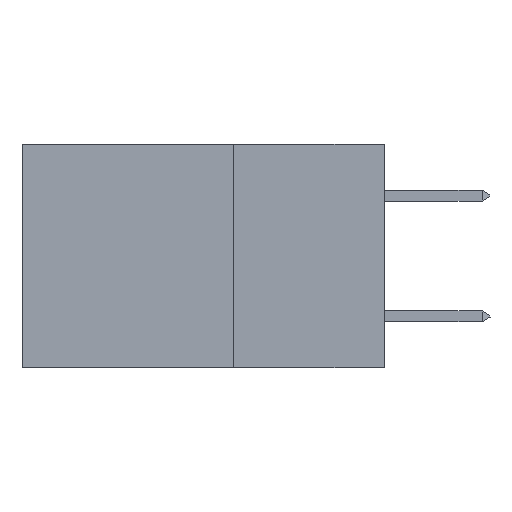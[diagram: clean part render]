
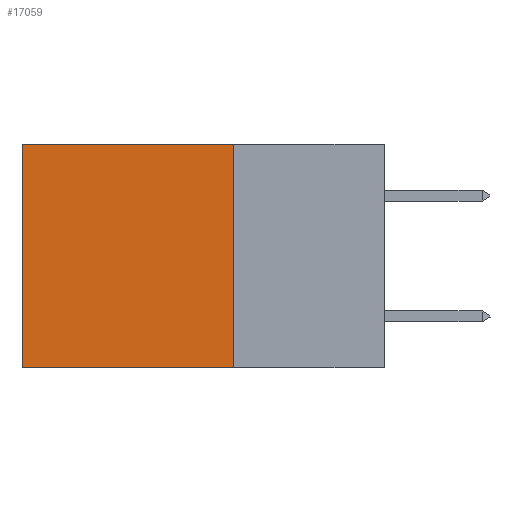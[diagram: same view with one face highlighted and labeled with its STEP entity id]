
A CAD part, left-side view. The second image highlights one B-rep face of the part: STEP entity #17059.
In plain terms, the highlighted planar face has unit normal (-1, 0, 0).
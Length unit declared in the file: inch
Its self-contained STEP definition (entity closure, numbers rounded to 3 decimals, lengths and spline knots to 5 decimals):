
#286 = VECTOR ( 'NONE', #23873, 39.37008 ) ;
#398 = CARTESIAN_POINT ( 'NONE',  ( 0.2875, 0.25, -0.37 ) ) ;
#1246 = CARTESIAN_POINT ( 'NONE',  ( 0.2875, 0.25, 0. ) ) ;
#1884 = VERTEX_POINT ( 'NONE', #398 ) ;
#2504 = EDGE_CURVE ( 'NONE', #1884, #13076, #17662, .T. ) ;
#3411 = DIRECTION ( 'NONE',  ( 0., 1., 0. ) ) ;
#3671 = DIRECTION ( 'NONE',  ( 1., 0., 0. ) ) ;
#3763 = DIRECTION ( 'NONE',  ( 0., 1., 0. ) ) ;
#6513 = EDGE_LOOP ( 'NONE', ( #12522, #27516, #12383, #24293 ) ) ;
#8481 = CARTESIAN_POINT ( 'NONE',  ( 0.2875, 0.6, 0. ) ) ;
#10147 = VECTOR ( 'NONE', #20184, 39.37008 ) ;
#12070 = CARTESIAN_POINT ( 'NONE',  ( 0.2875, 0.6, 0. ) ) ;
#12383 = ORIENTED_EDGE ( 'NONE', *, *, #24379, .F. ) ;
#12522 = ORIENTED_EDGE ( 'NONE', *, *, #20179, .T. ) ;
#13076 = VERTEX_POINT ( 'NONE', #23577 ) ;
#14999 = CARTESIAN_POINT ( 'NONE',  ( 0.2875, 0.25, 0. ) ) ;
#15160 = AXIS2_PLACEMENT_3D ( 'NONE', #26642, #3671, #21998 ) ;
#15726 = FACE_OUTER_BOUND ( 'NONE', #6513, .T. ) ;
#16596 = VECTOR ( 'NONE', #3411, 39.37008 ) ;
#17059 = ADVANCED_FACE ( 'NONE', ( #15726 ), #26049, .F. ) ;
#17540 = VERTEX_POINT ( 'NONE', #12070 ) ;
#17662 = LINE ( 'NONE', #26390, #16596 ) ;
#20179 = EDGE_CURVE ( 'NONE', #17540, #13076, #29206, .T. ) ;
#20184 = DIRECTION ( 'NONE',  ( 0., 0., -1. ) ) ;
#20940 = LINE ( 'NONE', #14999, #22746 ) ;
#20962 = CARTESIAN_POINT ( 'NONE',  ( 0.2875, 0.25, 0. ) ) ;
#21998 = DIRECTION ( 'NONE',  ( 0., 0., -1. ) ) ;
#22651 = LINE ( 'NONE', #20962, #286 ) ;
#22746 = VECTOR ( 'NONE', #3763, 39.37008 ) ;
#23577 = CARTESIAN_POINT ( 'NONE',  ( 0.2875, 0.6, -0.37 ) ) ;
#23873 = DIRECTION ( 'NONE',  ( 0., 0., -1. ) ) ;
#24293 = ORIENTED_EDGE ( 'NONE', *, *, #28311, .T. ) ;
#24379 = EDGE_CURVE ( 'NONE', #29576, #1884, #22651, .T. ) ;
#26049 = PLANE ( 'NONE',  #15160 ) ;
#26390 = CARTESIAN_POINT ( 'NONE',  ( 0.2875, 0.25, -0.37 ) ) ;
#26642 = CARTESIAN_POINT ( 'NONE',  ( 0.2875, 0.25, 0. ) ) ;
#27516 = ORIENTED_EDGE ( 'NONE', *, *, #2504, .F. ) ;
#28311 = EDGE_CURVE ( 'NONE', #29576, #17540, #20940, .T. ) ;
#29206 = LINE ( 'NONE', #8481, #10147 ) ;
#29576 = VERTEX_POINT ( 'NONE', #1246 ) ;
